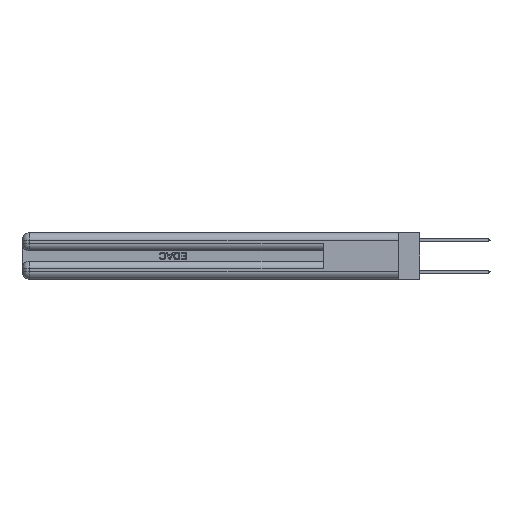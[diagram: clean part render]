
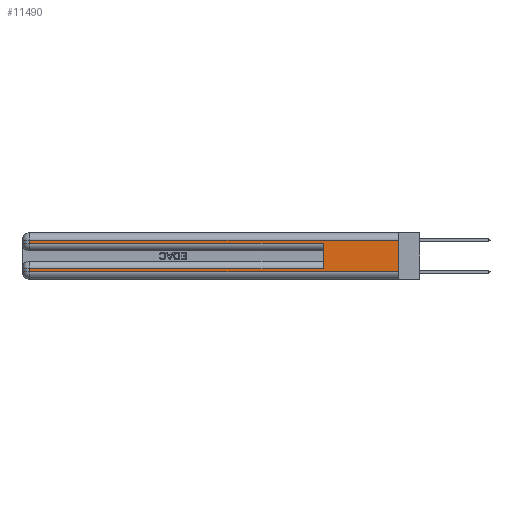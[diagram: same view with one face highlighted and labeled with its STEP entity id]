
A CAD part, left-side view. The second image highlights one B-rep face of the part: STEP entity #11490.
In plain terms, the highlighted planar face has unit normal (-1, 0, 0).
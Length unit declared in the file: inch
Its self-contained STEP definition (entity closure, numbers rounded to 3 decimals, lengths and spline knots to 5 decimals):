
#86 = CARTESIAN_POINT ( 'NONE',  ( 0., 0., 0.285 ) ) ;
#137 = ORIENTED_EDGE ( 'NONE', *, *, #22722, .T. ) ;
#648 = ORIENTED_EDGE ( 'NONE', *, *, #24123, .T. ) ;
#1053 = ORIENTED_EDGE ( 'NONE', *, *, #15145, .F. ) ;
#1652 = DIRECTION ( 'NONE',  ( 0., 0., -1. ) ) ;
#1834 = EDGE_CURVE ( 'NONE', #12933, #20850, #29570, .T. ) ;
#2039 = VERTEX_POINT ( 'NONE', #26007 ) ;
#2489 = EDGE_LOOP ( 'NONE', ( #4428, #8057, #14939, #648, #1053, #4068, #18375, #137 ) ) ;
#2679 = VERTEX_POINT ( 'NONE', #16384 ) ;
#2996 = CARTESIAN_POINT ( 'NONE',  ( 0., 2.94, 0.285 ) ) ;
#3087 = DIRECTION ( 'NONE',  ( 0., 1., 0. ) ) ;
#3212 = VERTEX_POINT ( 'NONE', #21859 ) ;
#3347 = VERTEX_POINT ( 'NONE', #2996 ) ;
#4068 = ORIENTED_EDGE ( 'NONE', *, *, #4702, .T. ) ;
#4428 = ORIENTED_EDGE ( 'NONE', *, *, #22049, .F. ) ;
#4702 = EDGE_CURVE ( 'NONE', #32885, #12933, #8132, .T. ) ;
#5493 = VECTOR ( 'NONE', #6686, 39.37008 ) ;
#6686 = DIRECTION ( 'NONE',  ( 0., 0., -1. ) ) ;
#6886 = LINE ( 'NONE', #14134, #25328 ) ;
#7549 = AXIS2_PLACEMENT_3D ( 'NONE', #7875, #18129, #13431 ) ;
#7875 = CARTESIAN_POINT ( 'NONE',  ( 0., 0., 0.37 ) ) ;
#8057 = ORIENTED_EDGE ( 'NONE', *, *, #30406, .T. ) ;
#8132 = LINE ( 'NONE', #31825, #32165 ) ;
#8158 = DIRECTION ( 'NONE',  ( 0., -1., 0. ) ) ;
#9340 = DIRECTION ( 'NONE',  ( 0., -1., 0. ) ) ;
#11236 = FACE_OUTER_BOUND ( 'NONE', #2489, .T. ) ;
#11249 = CARTESIAN_POINT ( 'NONE',  ( 0., 0., 0.37 ) ) ;
#11490 = ADVANCED_FACE ( 'NONE', ( #11236 ), #21473, .F. ) ;
#12933 = VERTEX_POINT ( 'NONE', #32620 ) ;
#13431 = DIRECTION ( 'NONE',  ( 0., 0., -1. ) ) ;
#13933 = DIRECTION ( 'NONE',  ( 0., 1., 0. ) ) ;
#13974 = DIRECTION ( 'NONE',  ( 0., 0., -1. ) ) ;
#14134 = CARTESIAN_POINT ( 'NONE',  ( 0., 2.94, 0.37 ) ) ;
#14230 = CARTESIAN_POINT ( 'NONE',  ( 0., 0.6, 0.145 ) ) ;
#14550 = CARTESIAN_POINT ( 'NONE',  ( 0., 0., 0.06 ) ) ;
#14939 = ORIENTED_EDGE ( 'NONE', *, *, #31691, .T. ) ;
#15047 = VERTEX_POINT ( 'NONE', #16106 ) ;
#15145 = EDGE_CURVE ( 'NONE', #32885, #2039, #29861, .T. ) ;
#16106 = CARTESIAN_POINT ( 'NONE',  ( 0., 0., 0.06 ) ) ;
#16384 = CARTESIAN_POINT ( 'NONE',  ( 0., 0., 0.31 ) ) ;
#17435 = CARTESIAN_POINT ( 'NONE',  ( 0., 2.94, 0.37 ) ) ;
#18129 = DIRECTION ( 'NONE',  ( 1., 0., 0. ) ) ;
#18375 = ORIENTED_EDGE ( 'NONE', *, *, #1834, .T. ) ;
#19929 = DIRECTION ( 'NONE',  ( 0., 0., 1. ) ) ;
#20233 = VECTOR ( 'NONE', #8158, 39.37008 ) ;
#20850 = VERTEX_POINT ( 'NONE', #32199 ) ;
#21212 = CARTESIAN_POINT ( 'NONE',  ( 0., 0.6, 0.085 ) ) ;
#21473 = PLANE ( 'NONE',  #7549 ) ;
#21747 = VECTOR ( 'NONE', #1652, 39.37008 ) ;
#21859 = CARTESIAN_POINT ( 'NONE',  ( 0., 2.94, 0.31 ) ) ;
#22049 = EDGE_CURVE ( 'NONE', #2679, #15047, #32250, .T. ) ;
#22722 = EDGE_CURVE ( 'NONE', #20850, #15047, #27637, .T. ) ;
#23098 = VECTOR ( 'NONE', #13933, 39.37008 ) ;
#23611 = LINE ( 'NONE', #86, #20233 ) ;
#24123 = EDGE_CURVE ( 'NONE', #3347, #2039, #23611, .T. ) ;
#24288 = VECTOR ( 'NONE', #19929, 39.37008 ) ;
#24331 = LINE ( 'NONE', #26696, #23098 ) ;
#25328 = VECTOR ( 'NONE', #13974, 39.37008 ) ;
#26007 = CARTESIAN_POINT ( 'NONE',  ( 0., 0.6, 0.285 ) ) ;
#26696 = CARTESIAN_POINT ( 'NONE',  ( 0., 0., 0.31 ) ) ;
#27150 = VECTOR ( 'NONE', #9340, 39.37008 ) ;
#27637 = LINE ( 'NONE', #14550, #27150 ) ;
#29570 = LINE ( 'NONE', #17435, #5493 ) ;
#29861 = LINE ( 'NONE', #14230, #24288 ) ;
#30406 = EDGE_CURVE ( 'NONE', #2679, #3212, #24331, .T. ) ;
#31691 = EDGE_CURVE ( 'NONE', #3212, #3347, #6886, .T. ) ;
#31825 = CARTESIAN_POINT ( 'NONE',  ( 0., 0., 0.085 ) ) ;
#32165 = VECTOR ( 'NONE', #3087, 39.37008 ) ;
#32199 = CARTESIAN_POINT ( 'NONE',  ( 0., 2.94, 0.06 ) ) ;
#32250 = LINE ( 'NONE', #11249, #21747 ) ;
#32620 = CARTESIAN_POINT ( 'NONE',  ( 0., 2.94, 0.085 ) ) ;
#32885 = VERTEX_POINT ( 'NONE', #21212 ) ;
